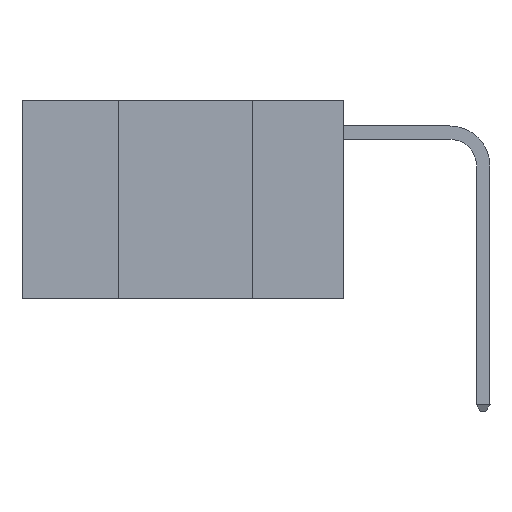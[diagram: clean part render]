
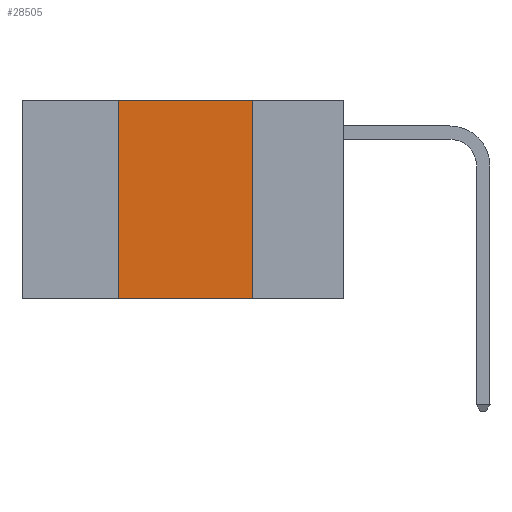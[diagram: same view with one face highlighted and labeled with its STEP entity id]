
A CAD part, left-side view. The second image highlights one B-rep face of the part: STEP entity #28505.
In plain terms, the highlighted planar face has unit normal (-1, 0, 0).
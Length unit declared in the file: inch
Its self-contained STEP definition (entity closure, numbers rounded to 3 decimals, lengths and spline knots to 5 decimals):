
#1828 = DIRECTION ( 'NONE',  ( 0., 0., -1. ) ) ;
#1961 = LINE ( 'NONE', #7924, #3470 ) ;
#2480 = DIRECTION ( 'NONE',  ( 0., 0., -1. ) ) ;
#3470 = VECTOR ( 'NONE', #10375, 39.37008 ) ;
#4161 = VECTOR ( 'NONE', #5444, 39.37008 ) ;
#5267 = ORIENTED_EDGE ( 'NONE', *, *, #15734, .F. ) ;
#5444 = DIRECTION ( 'NONE',  ( 0., -1., 0. ) ) ;
#5487 = LINE ( 'NONE', #17041, #30494 ) ;
#6625 = CARTESIAN_POINT ( 'NONE',  ( 0., 0.42, -0.37 ) ) ;
#7860 = VERTEX_POINT ( 'NONE', #6625 ) ;
#7924 = CARTESIAN_POINT ( 'NONE',  ( 0., 0.6, -0.37 ) ) ;
#8030 = DIRECTION ( 'NONE',  ( 0., 0., 1. ) ) ;
#9649 = ORIENTED_EDGE ( 'NONE', *, *, #17497, .T. ) ;
#9651 = EDGE_CURVE ( 'NONE', #26957, #16594, #5487, .T. ) ;
#9816 = LINE ( 'NONE', #22384, #4161 ) ;
#10375 = DIRECTION ( 'NONE',  ( 0., -1., 0. ) ) ;
#10556 = ORIENTED_EDGE ( 'NONE', *, *, #9651, .F. ) ;
#10761 = VECTOR ( 'NONE', #8030, 39.37008 ) ;
#13307 = EDGE_CURVE ( 'NONE', #26864, #26957, #9816, .T. ) ;
#13854 = PLANE ( 'NONE',  #15266 ) ;
#15266 = AXIS2_PLACEMENT_3D ( 'NONE', #23493, #16285, #1828 ) ;
#15734 = EDGE_CURVE ( 'NONE', #7860, #26864, #17202, .T. ) ;
#16285 = DIRECTION ( 'NONE',  ( 1., 0., 0. ) ) ;
#16594 = VERTEX_POINT ( 'NONE', #23975 ) ;
#17041 = CARTESIAN_POINT ( 'NONE',  ( 0., 0.17, 0. ) ) ;
#17202 = LINE ( 'NONE', #29888, #10761 ) ;
#17497 = EDGE_CURVE ( 'NONE', #7860, #16594, #1961, .T. ) ;
#20349 = EDGE_LOOP ( 'NONE', ( #10556, #30283, #5267, #9649 ) ) ;
#22384 = CARTESIAN_POINT ( 'NONE',  ( 0., 0.6, 0. ) ) ;
#23140 = CARTESIAN_POINT ( 'NONE',  ( 0., 0.42, 0. ) ) ;
#23493 = CARTESIAN_POINT ( 'NONE',  ( 0., 0.6, 0. ) ) ;
#23975 = CARTESIAN_POINT ( 'NONE',  ( 0., 0.17, -0.37 ) ) ;
#25137 = FACE_OUTER_BOUND ( 'NONE', #20349, .T. ) ;
#26864 = VERTEX_POINT ( 'NONE', #23140 ) ;
#26957 = VERTEX_POINT ( 'NONE', #30896 ) ;
#28505 = ADVANCED_FACE ( 'NONE', ( #25137 ), #13854, .F. ) ;
#29888 = CARTESIAN_POINT ( 'NONE',  ( 0., 0.42, 0. ) ) ;
#30283 = ORIENTED_EDGE ( 'NONE', *, *, #13307, .F. ) ;
#30494 = VECTOR ( 'NONE', #2480, 39.37008 ) ;
#30896 = CARTESIAN_POINT ( 'NONE',  ( 0., 0.17, 0. ) ) ;
